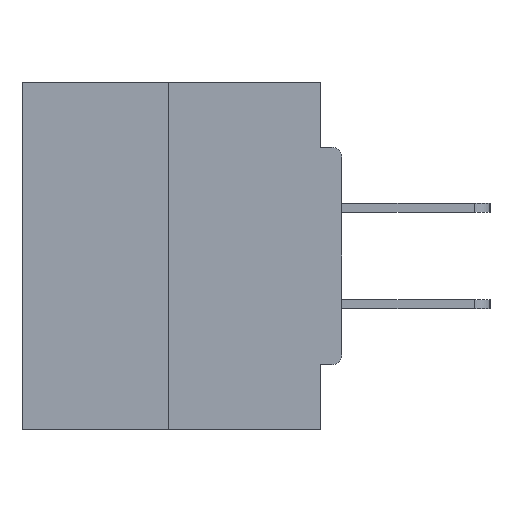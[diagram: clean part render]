
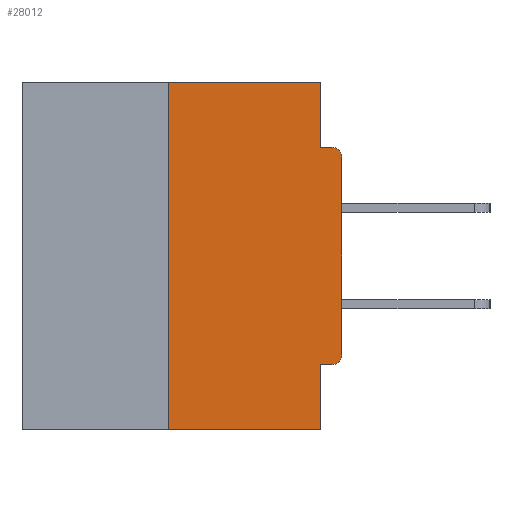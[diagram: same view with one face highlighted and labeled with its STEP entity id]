
A CAD part, left-side view. The second image highlights one B-rep face of the part: STEP entity #28012.
In plain terms, the highlighted planar face has unit normal (-1, 0, 0).
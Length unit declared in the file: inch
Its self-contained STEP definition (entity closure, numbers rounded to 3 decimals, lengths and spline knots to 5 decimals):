
#482 = ORIENTED_EDGE ( 'NONE', *, *, #4930, .T. ) ;
#1171 = VECTOR ( 'NONE', #28585, 39.37008 ) ;
#1256 = CARTESIAN_POINT ( 'NONE',  ( 0., 0.46, -0.5 ) ) ;
#2045 = EDGE_CURVE ( 'NONE', #23458, #22870, #10861, .T. ) ;
#2161 = CARTESIAN_POINT ( 'NONE',  ( 0., 0.031, -0.5 ) ) ;
#2627 = PLANE ( 'NONE',  #29159 ) ;
#2934 = EDGE_CURVE ( 'NONE', #10590, #19609, #27099, .T. ) ;
#3292 = ORIENTED_EDGE ( 'NONE', *, *, #11428, .F. ) ;
#4230 = EDGE_CURVE ( 'NONE', #10590, #28876, #12538, .T. ) ;
#4380 = CARTESIAN_POINT ( 'NONE',  ( 0., 0.25, -0.5 ) ) ;
#4930 = EDGE_CURVE ( 'NONE', #21613, #12244, #14137, .T. ) ;
#5127 = DIRECTION ( 'NONE',  ( -1., 0., 0. ) ) ;
#5304 = CARTESIAN_POINT ( 'NONE',  ( 0., 0.031, 0. ) ) ;
#5683 = CARTESIAN_POINT ( 'NONE',  ( 0., 0.015, -0.1085 ) ) ;
#6032 = CARTESIAN_POINT ( 'NONE',  ( 0., 0., 0. ) ) ;
#6266 = ORIENTED_EDGE ( 'NONE', *, *, #23390, .T. ) ;
#6896 = LINE ( 'NONE', #5304, #31135 ) ;
#6979 = EDGE_CURVE ( 'NONE', #18302, #23458, #6896, .T. ) ;
#7007 = DIRECTION ( 'NONE',  ( 0., 0., 1. ) ) ;
#7284 = ORIENTED_EDGE ( 'NONE', *, *, #4230, .T. ) ;
#7544 = CARTESIAN_POINT ( 'NONE',  ( 0., 0., -0.4065 ) ) ;
#8814 = EDGE_CURVE ( 'NONE', #20835, #28876, #33553, .T. ) ;
#9558 = CARTESIAN_POINT ( 'NONE',  ( 0., 0.031, 0. ) ) ;
#9719 = CARTESIAN_POINT ( 'NONE',  ( 0., 0.015, -0.4065 ) ) ;
#10245 = ORIENTED_EDGE ( 'NONE', *, *, #2045, .F. ) ;
#10590 = VERTEX_POINT ( 'NONE', #4380 ) ;
#10861 = LINE ( 'NONE', #30571, #33095 ) ;
#11380 = EDGE_CURVE ( 'NONE', #19609, #18302, #14567, .T. ) ;
#11428 = EDGE_CURVE ( 'NONE', #21613, #20835, #31726, .T. ) ;
#11658 = DIRECTION ( 'NONE',  ( 0., -1., 0. ) ) ;
#12244 = VERTEX_POINT ( 'NONE', #33493 ) ;
#12530 = ORIENTED_EDGE ( 'NONE', *, *, #8814, .F. ) ;
#12538 = LINE ( 'NONE', #1256, #31370 ) ;
#13358 = CARTESIAN_POINT ( 'NONE',  ( 0., 0.031, -0.4065 ) ) ;
#13478 = DIRECTION ( 'NONE',  ( -1., 0., 0. ) ) ;
#13824 = ORIENTED_EDGE ( 'NONE', *, *, #11380, .F. ) ;
#14063 = CARTESIAN_POINT ( 'NONE',  ( 0., 0.46, 0. ) ) ;
#14137 = CIRCLE ( 'NONE', #24493, 0.015 ) ;
#14567 = LINE ( 'NONE', #14063, #34320 ) ;
#15040 = CARTESIAN_POINT ( 'NONE',  ( 0., 0., -0.1085 ) ) ;
#15059 = ORIENTED_EDGE ( 'NONE', *, *, #6979, .F. ) ;
#15526 = CARTESIAN_POINT ( 'NONE',  ( 0., 0.015, -0.3915 ) ) ;
#16167 = DIRECTION ( 'NONE',  ( 0., 0., -1. ) ) ;
#16263 = CARTESIAN_POINT ( 'NONE',  ( 0., 0.25, 0. ) ) ;
#16851 = VECTOR ( 'NONE', #29751, 39.37008 ) ;
#17296 = AXIS2_PLACEMENT_3D ( 'NONE', #5683, #13478, #32497 ) ;
#17304 = EDGE_LOOP ( 'NONE', ( #13824, #26949, #7284, #12530, #3292, #482, #6266, #23170, #10245, #15059 ) ) ;
#17379 = DIRECTION ( 'NONE',  ( 0., -1., 0. ) ) ;
#18141 = EDGE_CURVE ( 'NONE', #26989, #22870, #19395, .T. ) ;
#18302 = VERTEX_POINT ( 'NONE', #9558 ) ;
#19395 = CIRCLE ( 'NONE', #17296, 0.015 ) ;
#19609 = VERTEX_POINT ( 'NONE', #16263 ) ;
#20835 = VERTEX_POINT ( 'NONE', #13358 ) ;
#20860 = DIRECTION ( 'NONE',  ( 0., 0., -1. ) ) ;
#21201 = VECTOR ( 'NONE', #7007, 39.37008 ) ;
#21613 = VERTEX_POINT ( 'NONE', #9719 ) ;
#22870 = VERTEX_POINT ( 'NONE', #32173 ) ;
#23029 = CARTESIAN_POINT ( 'NONE',  ( 0., 0.031, -0.0935 ) ) ;
#23170 = ORIENTED_EDGE ( 'NONE', *, *, #18141, .T. ) ;
#23390 = EDGE_CURVE ( 'NONE', #12244, #26989, #31105, .T. ) ;
#23458 = VERTEX_POINT ( 'NONE', #23029 ) ;
#23925 = DIRECTION ( 'NONE',  ( 0., 0., -1. ) ) ;
#23928 = DIRECTION ( 'NONE',  ( 0., 0., -1. ) ) ;
#24060 = FACE_OUTER_BOUND ( 'NONE', #17304, .T. ) ;
#24493 = AXIS2_PLACEMENT_3D ( 'NONE', #15526, #5127, #23928 ) ;
#25077 = CARTESIAN_POINT ( 'NONE',  ( 0., 0.031, -0.5 ) ) ;
#26949 = ORIENTED_EDGE ( 'NONE', *, *, #2934, .F. ) ;
#26960 = CARTESIAN_POINT ( 'NONE',  ( 0., 0.46, 0. ) ) ;
#26989 = VERTEX_POINT ( 'NONE', #15040 ) ;
#27099 = LINE ( 'NONE', #33615, #21201 ) ;
#28012 = ADVANCED_FACE ( 'NONE', ( #24060 ), #2627, .F. ) ;
#28585 = DIRECTION ( 'NONE',  ( 0., 1., 0. ) ) ;
#28876 = VERTEX_POINT ( 'NONE', #25077 ) ;
#29159 = AXIS2_PLACEMENT_3D ( 'NONE', #26960, #29544, #23925 ) ;
#29544 = DIRECTION ( 'NONE',  ( 1., 0., 0. ) ) ;
#29751 = DIRECTION ( 'NONE',  ( 0., 0., 1. ) ) ;
#30571 = CARTESIAN_POINT ( 'NONE',  ( 0., 0., -0.0935 ) ) ;
#31105 = LINE ( 'NONE', #6032, #16851 ) ;
#31135 = VECTOR ( 'NONE', #16167, 39.37008 ) ;
#31370 = VECTOR ( 'NONE', #17379, 39.37008 ) ;
#31726 = LINE ( 'NONE', #7544, #1171 ) ;
#32173 = CARTESIAN_POINT ( 'NONE',  ( 0., 0.015, -0.0935 ) ) ;
#32497 = DIRECTION ( 'NONE',  ( 0., 0., -1. ) ) ;
#32832 = DIRECTION ( 'NONE',  ( 0., -1., 0. ) ) ;
#33095 = VECTOR ( 'NONE', #32832, 39.37008 ) ;
#33153 = VECTOR ( 'NONE', #20860, 39.37008 ) ;
#33493 = CARTESIAN_POINT ( 'NONE',  ( 0., 0., -0.3915 ) ) ;
#33553 = LINE ( 'NONE', #2161, #33153 ) ;
#33615 = CARTESIAN_POINT ( 'NONE',  ( 0., 0.25, 0. ) ) ;
#34320 = VECTOR ( 'NONE', #11658, 39.37008 ) ;
